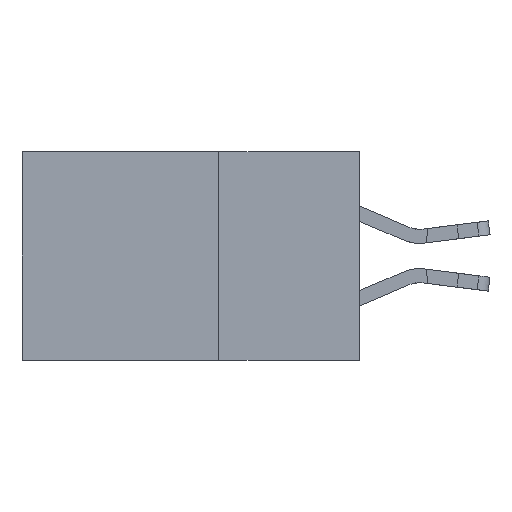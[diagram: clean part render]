
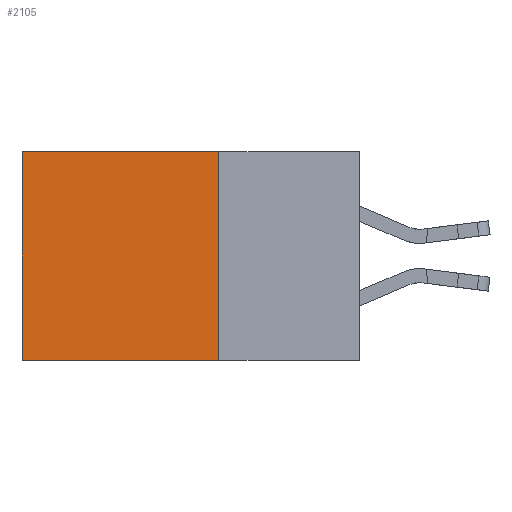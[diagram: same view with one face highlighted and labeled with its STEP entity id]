
A CAD part, left-side view. The second image highlights one B-rep face of the part: STEP entity #2105.
In plain terms, the highlighted planar face has unit normal (-1, 0, 0).
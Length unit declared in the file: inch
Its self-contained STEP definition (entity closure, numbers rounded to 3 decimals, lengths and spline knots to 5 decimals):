
#826 = VERTEX_POINT ( 'NONE', #6867 ) ;
#1104 = CARTESIAN_POINT ( 'NONE',  ( 0.2875, 0.6, 0. ) ) ;
#1697 = LINE ( 'NONE', #18060, #2396 ) ;
#2105 = ADVANCED_FACE ( 'NONE', ( #3517 ), #19651, .F. ) ;
#2285 = CARTESIAN_POINT ( 'NONE',  ( 0.2875, 0.25, 0. ) ) ;
#2396 = VECTOR ( 'NONE', #13856, 39.37008 ) ;
#3517 = FACE_OUTER_BOUND ( 'NONE', #21314, .T. ) ;
#4615 = VERTEX_POINT ( 'NONE', #19760 ) ;
#5171 = VECTOR ( 'NONE', #13181, 39.37008 ) ;
#5536 = VERTEX_POINT ( 'NONE', #16543 ) ;
#5661 = VERTEX_POINT ( 'NONE', #12619 ) ;
#6804 = DIRECTION ( 'NONE',  ( 1., 0., 0. ) ) ;
#6867 = CARTESIAN_POINT ( 'NONE',  ( 0.2875, 0.6, -0.37 ) ) ;
#8305 = EDGE_CURVE ( 'NONE', #5661, #5536, #23862, .T. ) ;
#9857 = ORIENTED_EDGE ( 'NONE', *, *, #20247, .T. ) ;
#11614 = LINE ( 'NONE', #25940, #5171 ) ;
#11869 = EDGE_CURVE ( 'NONE', #5536, #826, #1697, .T. ) ;
#12071 = DIRECTION ( 'NONE',  ( 0., 0., -1. ) ) ;
#12531 = VECTOR ( 'NONE', #20545, 39.37008 ) ;
#12619 = CARTESIAN_POINT ( 'NONE',  ( 0.2875, 0.25, 0. ) ) ;
#12752 = ORIENTED_EDGE ( 'NONE', *, *, #23532, .T. ) ;
#13181 = DIRECTION ( 'NONE',  ( 0., 1., 0. ) ) ;
#13856 = DIRECTION ( 'NONE',  ( 0., 1., 0. ) ) ;
#16125 = LINE ( 'NONE', #1104, #26762 ) ;
#16543 = CARTESIAN_POINT ( 'NONE',  ( 0.2875, 0.25, -0.37 ) ) ;
#17991 = ORIENTED_EDGE ( 'NONE', *, *, #11869, .F. ) ;
#18060 = CARTESIAN_POINT ( 'NONE',  ( 0.2875, 0.25, -0.37 ) ) ;
#18399 = CARTESIAN_POINT ( 'NONE',  ( 0.2875, 0.25, 0. ) ) ;
#19651 = PLANE ( 'NONE',  #27030 ) ;
#19760 = CARTESIAN_POINT ( 'NONE',  ( 0.2875, 0.6, 0. ) ) ;
#20247 = EDGE_CURVE ( 'NONE', #5661, #4615, #11614, .T. ) ;
#20545 = DIRECTION ( 'NONE',  ( 0., 0., -1. ) ) ;
#21314 = EDGE_LOOP ( 'NONE', ( #12752, #17991, #22888, #9857 ) ) ;
#21778 = DIRECTION ( 'NONE',  ( 0., 0., -1. ) ) ;
#22888 = ORIENTED_EDGE ( 'NONE', *, *, #8305, .F. ) ;
#23532 = EDGE_CURVE ( 'NONE', #4615, #826, #16125, .T. ) ;
#23862 = LINE ( 'NONE', #18399, #12531 ) ;
#25940 = CARTESIAN_POINT ( 'NONE',  ( 0.2875, 0.25, 0. ) ) ;
#26762 = VECTOR ( 'NONE', #12071, 39.37008 ) ;
#27030 = AXIS2_PLACEMENT_3D ( 'NONE', #2285, #6804, #21778 ) ;
